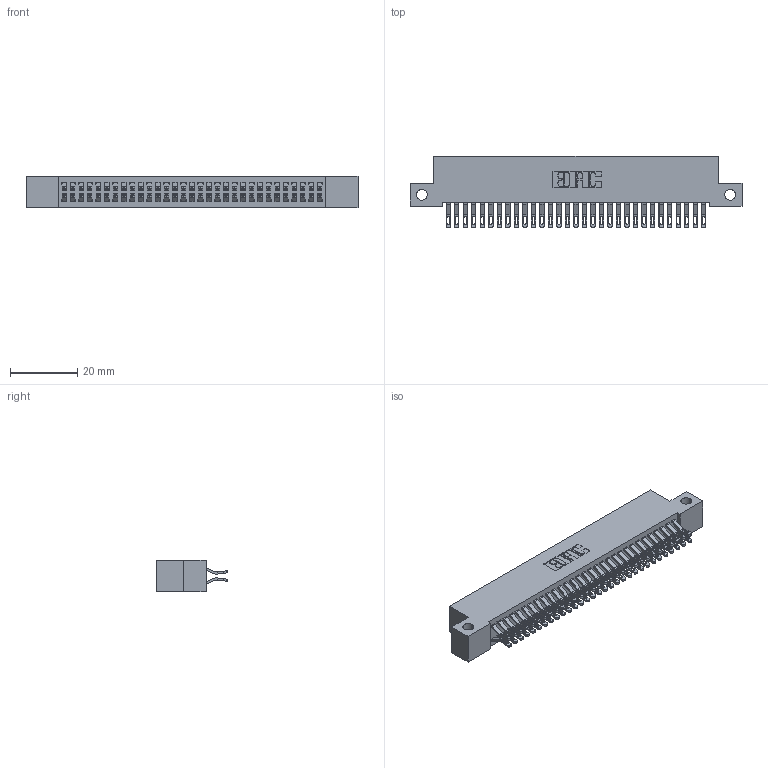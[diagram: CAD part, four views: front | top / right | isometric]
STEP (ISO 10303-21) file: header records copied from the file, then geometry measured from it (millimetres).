
FILE_DESCRIPTION (( 'STEP AP203' ), '1' );
FILE_NAME ('342-062-555-212.STEP', '2019-10-03T14:01:38', ( '' ), ( '' ), 'SwSTEP 2.0', 'SolidWorks 2016', '' );
FILE_SCHEMA (( 'CONFIG_CONTROL_DESIGN' ));
Length unit declared in the file: inch
Products named in the file (3): 342 Part_Side Mount; 345-292-001_555 Tail; 342-062-555-212
Assembly tree (63 placements, depth 2):
  342-062-555-212
    342 Part_Side Mount
    345-292-001_555 Tail  x62
Bounding box: 99.06 x 21.47 x 9.4 mm (x, y, z)
Volume: 8946.8 mm3; surface area: 14732.3 mm2
Topology: 63 solids, 63 shells, 3706 faces, 11645 edges, 7762 vertices
Faces by surface type: plane 2174, cylinder 1532
Entity records: 21563 total; most frequent: CARTESIAN_POINT 3620, ORIENTED_EDGE 3526, DIRECTION 3083, EDGE_CURVE 1763, LINE 1615, VECTOR 1615, VERTEX_POINT 1174, AXIS2_PLACEMENT_3D 734
